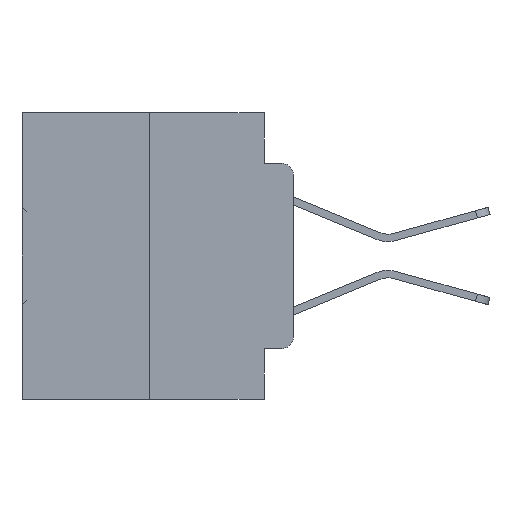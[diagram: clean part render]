
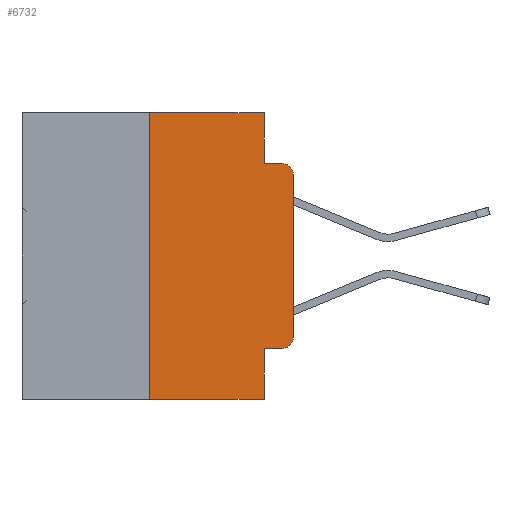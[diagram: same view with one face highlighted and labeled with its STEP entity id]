
A CAD part, left-side view. The second image highlights one B-rep face of the part: STEP entity #6732.
In plain terms, the highlighted planar face has unit normal (-1, 0, 0).
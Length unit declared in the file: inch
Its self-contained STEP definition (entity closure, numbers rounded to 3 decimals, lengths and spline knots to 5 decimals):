
#701 = CARTESIAN_POINT ( 'NONE',  ( 0., 0.473, -0.5 ) ) ;
#1253 = PLANE ( 'NONE',  #2449 ) ;
#1269 = DIRECTION ( 'NONE',  ( -1., 0., 0. ) ) ;
#2179 = EDGE_CURVE ( 'NONE', #18007, #15870, #5133, .T. ) ;
#2403 = LINE ( 'NONE', #14836, #30684 ) ;
#2449 = AXIS2_PLACEMENT_3D ( 'NONE', #4013, #31222, #25591 ) ;
#3228 = CIRCLE ( 'NONE', #28405, 0.02 ) ;
#4013 = CARTESIAN_POINT ( 'NONE',  ( 0., 0.473, 0. ) ) ;
#4468 = CARTESIAN_POINT ( 'NONE',  ( 0., 0.02, -0.3915 ) ) ;
#4679 = VECTOR ( 'NONE', #35219, 39.37008 ) ;
#4698 = ORIENTED_EDGE ( 'NONE', *, *, #8297, .T. ) ;
#5133 = LINE ( 'NONE', #35585, #4679 ) ;
#5189 = LINE ( 'NONE', #20319, #17153 ) ;
#5652 = ORIENTED_EDGE ( 'NONE', *, *, #8357, .F. ) ;
#6329 = DIRECTION ( 'NONE',  ( 0., 0., 1. ) ) ;
#6598 = DIRECTION ( 'NONE',  ( 0., 0., -1. ) ) ;
#6627 = LINE ( 'NONE', #14787, #27196 ) ;
#6732 = ADVANCED_FACE ( 'NONE', ( #28205 ), #1253, .F. ) ;
#7231 = CARTESIAN_POINT ( 'NONE',  ( 0., 0.02, -0.4115 ) ) ;
#7479 = DIRECTION ( 'NONE',  ( 0., -1., 0. ) ) ;
#7597 = CARTESIAN_POINT ( 'NONE',  ( 0., 0.473, 0. ) ) ;
#8297 = EDGE_CURVE ( 'NONE', #10917, #28262, #3228, .T. ) ;
#8357 = EDGE_CURVE ( 'NONE', #18962, #34056, #19056, .T. ) ;
#8935 = LINE ( 'NONE', #10180, #26983 ) ;
#9876 = ORIENTED_EDGE ( 'NONE', *, *, #26686, .F. ) ;
#10180 = CARTESIAN_POINT ( 'NONE',  ( 0., 0., 0. ) ) ;
#10410 = CARTESIAN_POINT ( 'NONE',  ( 0., 0.25, -0.5 ) ) ;
#10416 = ORIENTED_EDGE ( 'NONE', *, *, #19735, .T. ) ;
#10695 = VERTEX_POINT ( 'NONE', #10893 ) ;
#10893 = CARTESIAN_POINT ( 'NONE',  ( 0., 0., -0.3915 ) ) ;
#10917 = VERTEX_POINT ( 'NONE', #24134 ) ;
#12522 = CARTESIAN_POINT ( 'NONE',  ( 0., 0.051, -0.0885 ) ) ;
#12875 = DIRECTION ( 'NONE',  ( 0., 0., -1. ) ) ;
#14030 = VECTOR ( 'NONE', #15742, 39.37008 ) ;
#14664 = ORIENTED_EDGE ( 'NONE', *, *, #33488, .T. ) ;
#14787 = CARTESIAN_POINT ( 'NONE',  ( 0., 0.25, 0. ) ) ;
#14836 = CARTESIAN_POINT ( 'NONE',  ( 0., 0.051, 0. ) ) ;
#15140 = CARTESIAN_POINT ( 'NONE',  ( 0., 0.02, -0.1085 ) ) ;
#15612 = CARTESIAN_POINT ( 'NONE',  ( 0., 0.051, 0. ) ) ;
#15742 = DIRECTION ( 'NONE',  ( 0., -1., 0. ) ) ;
#15870 = VERTEX_POINT ( 'NONE', #7231 ) ;
#17040 = LINE ( 'NONE', #701, #35161 ) ;
#17153 = VECTOR ( 'NONE', #7479, 39.37008 ) ;
#17330 = VECTOR ( 'NONE', #12875, 39.37008 ) ;
#17712 = ORIENTED_EDGE ( 'NONE', *, *, #19231, .T. ) ;
#17736 = AXIS2_PLACEMENT_3D ( 'NONE', #4468, #23608, #34589 ) ;
#18007 = VERTEX_POINT ( 'NONE', #22735 ) ;
#18334 = CARTESIAN_POINT ( 'NONE',  ( 0., 0.25, 0. ) ) ;
#18962 = VERTEX_POINT ( 'NONE', #29600 ) ;
#19056 = LINE ( 'NONE', #15612, #17330 ) ;
#19231 = EDGE_CURVE ( 'NONE', #15870, #10695, #21766, .T. ) ;
#19735 = EDGE_CURVE ( 'NONE', #22950, #32249, #17040, .T. ) ;
#19940 = ORIENTED_EDGE ( 'NONE', *, *, #23999, .F. ) ;
#20319 = CARTESIAN_POINT ( 'NONE',  ( 0., 0.051, -0.0885 ) ) ;
#20402 = ORIENTED_EDGE ( 'NONE', *, *, #2179, .T. ) ;
#20469 = LINE ( 'NONE', #7597, #14030 ) ;
#21766 = CIRCLE ( 'NONE', #17736, 0.02 ) ;
#22735 = CARTESIAN_POINT ( 'NONE',  ( 0., 0.051, -0.4115 ) ) ;
#22950 = VERTEX_POINT ( 'NONE', #10410 ) ;
#22990 = ORIENTED_EDGE ( 'NONE', *, *, #29032, .F. ) ;
#23608 = DIRECTION ( 'NONE',  ( -1., 0., 0. ) ) ;
#23999 = EDGE_CURVE ( 'NONE', #18007, #32249, #2403, .T. ) ;
#24134 = CARTESIAN_POINT ( 'NONE',  ( 0., 0., -0.1085 ) ) ;
#24173 = DIRECTION ( 'NONE',  ( 0., 0., 1. ) ) ;
#24209 = VERTEX_POINT ( 'NONE', #18334 ) ;
#25591 = DIRECTION ( 'NONE',  ( 0., 0., -1. ) ) ;
#26609 = EDGE_LOOP ( 'NONE', ( #14664, #4698, #33092, #5652, #9876, #22990, #10416, #19940, #20402, #17712 ) ) ;
#26686 = EDGE_CURVE ( 'NONE', #24209, #18962, #20469, .T. ) ;
#26983 = VECTOR ( 'NONE', #24173, 39.37008 ) ;
#27196 = VECTOR ( 'NONE', #6329, 39.37008 ) ;
#27249 = CARTESIAN_POINT ( 'NONE',  ( 0., 0.051, -0.5 ) ) ;
#28205 = FACE_OUTER_BOUND ( 'NONE', #26609, .T. ) ;
#28262 = VERTEX_POINT ( 'NONE', #28749 ) ;
#28381 = DIRECTION ( 'NONE',  ( 0., -1., 0. ) ) ;
#28405 = AXIS2_PLACEMENT_3D ( 'NONE', #15140, #1269, #28699 ) ;
#28699 = DIRECTION ( 'NONE',  ( 0., 0., -1. ) ) ;
#28749 = CARTESIAN_POINT ( 'NONE',  ( 0., 0.02, -0.0885 ) ) ;
#29032 = EDGE_CURVE ( 'NONE', #22950, #24209, #6627, .T. ) ;
#29600 = CARTESIAN_POINT ( 'NONE',  ( 0., 0.051, 0. ) ) ;
#30684 = VECTOR ( 'NONE', #6598, 39.37008 ) ;
#31222 = DIRECTION ( 'NONE',  ( 1., 0., 0. ) ) ;
#32022 = EDGE_CURVE ( 'NONE', #34056, #28262, #5189, .T. ) ;
#32249 = VERTEX_POINT ( 'NONE', #27249 ) ;
#33092 = ORIENTED_EDGE ( 'NONE', *, *, #32022, .F. ) ;
#33488 = EDGE_CURVE ( 'NONE', #10695, #10917, #8935, .T. ) ;
#34056 = VERTEX_POINT ( 'NONE', #12522 ) ;
#34589 = DIRECTION ( 'NONE',  ( 0., 0., -1. ) ) ;
#35161 = VECTOR ( 'NONE', #28381, 39.37008 ) ;
#35219 = DIRECTION ( 'NONE',  ( 0., -1., 0. ) ) ;
#35585 = CARTESIAN_POINT ( 'NONE',  ( 0., 0.051, -0.4115 ) ) ;
